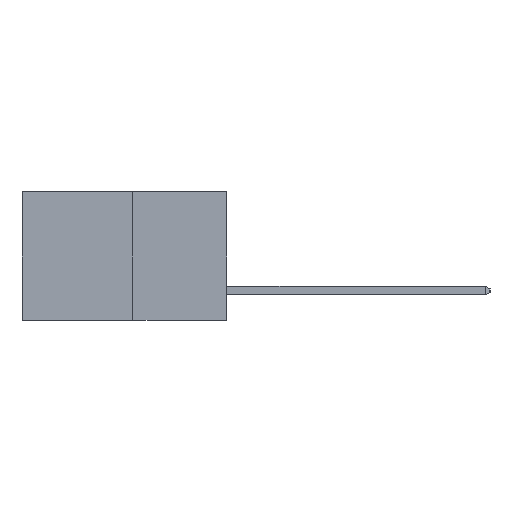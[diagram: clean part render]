
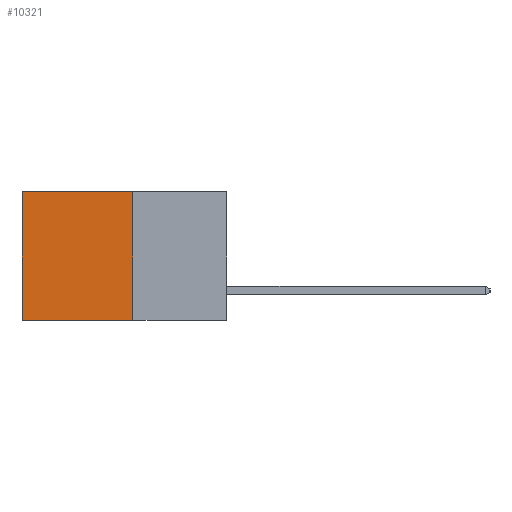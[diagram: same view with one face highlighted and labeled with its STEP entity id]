
A CAD part, left-side view. The second image highlights one B-rep face of the part: STEP entity #10321.
In plain terms, the highlighted planar face has unit normal (-1, 0, 0).
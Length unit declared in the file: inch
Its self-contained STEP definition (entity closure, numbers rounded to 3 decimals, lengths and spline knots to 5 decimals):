
#212 = VECTOR ( 'NONE', #8392, 39.37008 ) ;
#281 = VECTOR ( 'NONE', #2563, 39.37008 ) ;
#329 = CARTESIAN_POINT ( 'NONE',  ( 0.277, 0.59, -0.37 ) ) ;
#562 = CARTESIAN_POINT ( 'NONE',  ( 0.277, 0.27, -0.37 ) ) ;
#591 = VERTEX_POINT ( 'NONE', #10338 ) ;
#641 = ORIENTED_EDGE ( 'NONE', *, *, #7819, .T. ) ;
#863 = VECTOR ( 'NONE', #11759, 39.37008 ) ;
#1478 = CARTESIAN_POINT ( 'NONE',  ( 0.277, 0.27, -0.37 ) ) ;
#2185 = VERTEX_POINT ( 'NONE', #5189 ) ;
#2563 = DIRECTION ( 'NONE',  ( 0., 1., 0. ) ) ;
#2709 = ORIENTED_EDGE ( 'NONE', *, *, #10357, .T. ) ;
#2996 = LINE ( 'NONE', #6461, #281 ) ;
#3020 = ORIENTED_EDGE ( 'NONE', *, *, #7151, .F. ) ;
#3644 = FACE_OUTER_BOUND ( 'NONE', #5857, .T. ) ;
#5189 = CARTESIAN_POINT ( 'NONE',  ( 0.277, 0.27, 0. ) ) ;
#5191 = VECTOR ( 'NONE', #9564, 39.37008 ) ;
#5230 = AXIS2_PLACEMENT_3D ( 'NONE', #1478, #11900, #6418 ) ;
#5541 = LINE ( 'NONE', #10927, #212 ) ;
#5857 = EDGE_LOOP ( 'NONE', ( #641, #10592, #3020, #2709 ) ) ;
#6418 = DIRECTION ( 'NONE',  ( 0., 0., -1. ) ) ;
#6461 = CARTESIAN_POINT ( 'NONE',  ( 0.277, 0.27, 0. ) ) ;
#6716 = VERTEX_POINT ( 'NONE', #562 ) ;
#7151 = EDGE_CURVE ( 'NONE', #2185, #6716, #8314, .T. ) ;
#7688 = LINE ( 'NONE', #9639, #5191 ) ;
#7819 = EDGE_CURVE ( 'NONE', #591, #10231, #5541, .T. ) ;
#8314 = LINE ( 'NONE', #11716, #863 ) ;
#8392 = DIRECTION ( 'NONE',  ( 0., 0., -1. ) ) ;
#9067 = EDGE_CURVE ( 'NONE', #6716, #10231, #7688, .T. ) ;
#9564 = DIRECTION ( 'NONE',  ( 0., 1., 0. ) ) ;
#9639 = CARTESIAN_POINT ( 'NONE',  ( 0.277, 0.27, -0.37 ) ) ;
#10096 = PLANE ( 'NONE',  #5230 ) ;
#10231 = VERTEX_POINT ( 'NONE', #329 ) ;
#10321 = ADVANCED_FACE ( 'NONE', ( #3644 ), #10096, .F. ) ;
#10338 = CARTESIAN_POINT ( 'NONE',  ( 0.277, 0.59, 0. ) ) ;
#10357 = EDGE_CURVE ( 'NONE', #2185, #591, #2996, .T. ) ;
#10592 = ORIENTED_EDGE ( 'NONE', *, *, #9067, .F. ) ;
#10927 = CARTESIAN_POINT ( 'NONE',  ( 0.277, 0.59, -0.37 ) ) ;
#11716 = CARTESIAN_POINT ( 'NONE',  ( 0.277, 0.27, -0.37 ) ) ;
#11759 = DIRECTION ( 'NONE',  ( 0., 0., -1. ) ) ;
#11900 = DIRECTION ( 'NONE',  ( 1., 0., 0. ) ) ;
